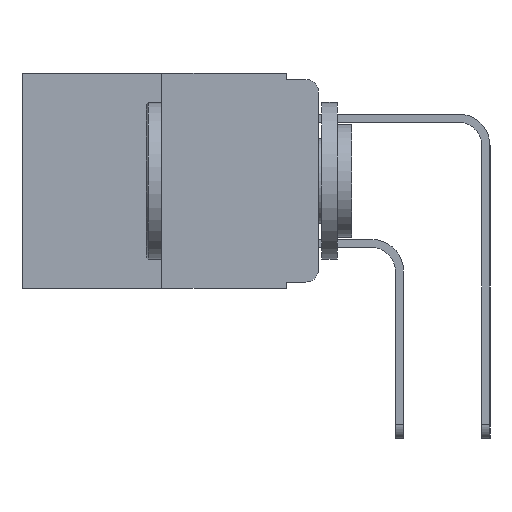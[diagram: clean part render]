
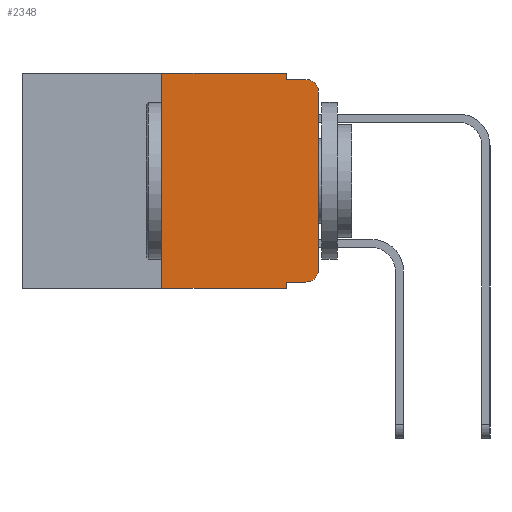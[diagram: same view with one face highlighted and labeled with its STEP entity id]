
A CAD part, left-side view. The second image highlights one B-rep face of the part: STEP entity #2348.
In plain terms, the highlighted planar face has unit normal (-1, 0, 0).
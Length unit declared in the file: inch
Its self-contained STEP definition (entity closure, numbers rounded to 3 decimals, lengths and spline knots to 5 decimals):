
#75 = ORIENTED_EDGE ( 'NONE', *, *, #12606, .F. ) ;
#532 = EDGE_CURVE ( 'NONE', #815, #10039, #12461, .T. ) ;
#646 = LINE ( 'NONE', #3511, #3547 ) ;
#777 = EDGE_CURVE ( 'NONE', #12841, #6741, #6242, .T. ) ;
#815 = VERTEX_POINT ( 'NONE', #12275 ) ;
#880 = AXIS2_PLACEMENT_3D ( 'NONE', #8151, #14173, #3209 ) ;
#946 = VECTOR ( 'NONE', #3475, 39.37008 ) ;
#975 = EDGE_LOOP ( 'NONE', ( #2216, #3295, #4586, #3999, #10049, #75, #2574, #1581, #1794, #2569 ) ) ;
#1115 = VERTEX_POINT ( 'NONE', #10265 ) ;
#1581 = ORIENTED_EDGE ( 'NONE', *, *, #7851, .F. ) ;
#1792 = CARTESIAN_POINT ( 'NONE',  ( 0., 0., -0.03 ) ) ;
#1794 = ORIENTED_EDGE ( 'NONE', *, *, #4811, .T. ) ;
#2216 = ORIENTED_EDGE ( 'NONE', *, *, #4131, .T. ) ;
#2348 = ADVANCED_FACE ( 'NONE', ( #10255 ), #11545, .F. ) ;
#2543 = CARTESIAN_POINT ( 'NONE',  ( 0., 0.051, -0.01 ) ) ;
#2569 = ORIENTED_EDGE ( 'NONE', *, *, #777, .T. ) ;
#2574 = ORIENTED_EDGE ( 'NONE', *, *, #11036, .T. ) ;
#2703 = VERTEX_POINT ( 'NONE', #3738 ) ;
#3000 = CARTESIAN_POINT ( 'NONE',  ( 0., 0.02, -0.313 ) ) ;
#3032 = DIRECTION ( 'NONE',  ( 0., 0., -1. ) ) ;
#3209 = DIRECTION ( 'NONE',  ( 0., 0., -1. ) ) ;
#3295 = ORIENTED_EDGE ( 'NONE', *, *, #5646, .T. ) ;
#3426 = VECTOR ( 'NONE', #4190, 39.37008 ) ;
#3443 = EDGE_CURVE ( 'NONE', #2703, #815, #9043, .T. ) ;
#3475 = DIRECTION ( 'NONE',  ( 0., 0., 1. ) ) ;
#3511 = CARTESIAN_POINT ( 'NONE',  ( 0., 0.473, 0. ) ) ;
#3547 = VECTOR ( 'NONE', #6862, 39.37008 ) ;
#3738 = CARTESIAN_POINT ( 'NONE',  ( 0., 0.051, 0. ) ) ;
#3834 = LINE ( 'NONE', #11164, #946 ) ;
#3999 = ORIENTED_EDGE ( 'NONE', *, *, #3443, .F. ) ;
#4131 = EDGE_CURVE ( 'NONE', #6741, #4433, #3834, .T. ) ;
#4190 = DIRECTION ( 'NONE',  ( 0., -1., 0. ) ) ;
#4214 = LINE ( 'NONE', #7473, #9705 ) ;
#4407 = AXIS2_PLACEMENT_3D ( 'NONE', #3000, #5075, #5576 ) ;
#4433 = VERTEX_POINT ( 'NONE', #1792 ) ;
#4586 = ORIENTED_EDGE ( 'NONE', *, *, #532, .F. ) ;
#4811 = EDGE_CURVE ( 'NONE', #12485, #12841, #6461, .T. ) ;
#4898 = CARTESIAN_POINT ( 'NONE',  ( 0., 0.051, -0.333 ) ) ;
#5075 = DIRECTION ( 'NONE',  ( -1., 0., 0. ) ) ;
#5100 = CARTESIAN_POINT ( 'NONE',  ( 0., 0.473, -0.343 ) ) ;
#5145 = VERTEX_POINT ( 'NONE', #11677 ) ;
#5342 = CARTESIAN_POINT ( 'NONE',  ( 0., 0.02, -0.333 ) ) ;
#5576 = DIRECTION ( 'NONE',  ( 0., 0., -1. ) ) ;
#5646 = EDGE_CURVE ( 'NONE', #4433, #10039, #8269, .T. ) ;
#6099 = CARTESIAN_POINT ( 'NONE',  ( 0., 0.25, -0.343 ) ) ;
#6230 = DIRECTION ( 'NONE',  ( -1., 0., 0. ) ) ;
#6233 = DIRECTION ( 'NONE',  ( 0., -1., 0. ) ) ;
#6242 = CIRCLE ( 'NONE', #4407, 0.02 ) ;
#6249 = LINE ( 'NONE', #5100, #11652 ) ;
#6461 = LINE ( 'NONE', #10736, #3426 ) ;
#6701 = EDGE_CURVE ( 'NONE', #5145, #2703, #646, .T. ) ;
#6741 = VERTEX_POINT ( 'NONE', #10165 ) ;
#6756 = VECTOR ( 'NONE', #7718, 39.37008 ) ;
#6862 = DIRECTION ( 'NONE',  ( 0., -1., 0. ) ) ;
#7215 = LINE ( 'NONE', #13698, #10089 ) ;
#7473 = CARTESIAN_POINT ( 'NONE',  ( 0., 0.051, 0. ) ) ;
#7718 = DIRECTION ( 'NONE',  ( 0., -1., 0. ) ) ;
#7851 = EDGE_CURVE ( 'NONE', #12485, #1115, #4214, .T. ) ;
#8151 = CARTESIAN_POINT ( 'NONE',  ( 0., 0.473, 0. ) ) ;
#8269 = CIRCLE ( 'NONE', #12304, 0.02 ) ;
#8704 = VECTOR ( 'NONE', #3032, 39.37008 ) ;
#9043 = LINE ( 'NONE', #10776, #8704 ) ;
#9705 = VECTOR ( 'NONE', #12802, 39.37008 ) ;
#10039 = VERTEX_POINT ( 'NONE', #11450 ) ;
#10049 = ORIENTED_EDGE ( 'NONE', *, *, #6701, .F. ) ;
#10089 = VECTOR ( 'NONE', #10521, 39.37008 ) ;
#10165 = CARTESIAN_POINT ( 'NONE',  ( 0., 0., -0.313 ) ) ;
#10255 = FACE_OUTER_BOUND ( 'NONE', #975, .T. ) ;
#10265 = CARTESIAN_POINT ( 'NONE',  ( 0., 0.051, -0.343 ) ) ;
#10521 = DIRECTION ( 'NONE',  ( 0., 0., 1. ) ) ;
#10736 = CARTESIAN_POINT ( 'NONE',  ( 0., 0.051, -0.333 ) ) ;
#10776 = CARTESIAN_POINT ( 'NONE',  ( 0., 0.051, 0. ) ) ;
#11036 = EDGE_CURVE ( 'NONE', #11698, #1115, #6249, .T. ) ;
#11164 = CARTESIAN_POINT ( 'NONE',  ( 0., 0., 0. ) ) ;
#11450 = CARTESIAN_POINT ( 'NONE',  ( 0., 0.02, -0.01 ) ) ;
#11545 = PLANE ( 'NONE',  #880 ) ;
#11652 = VECTOR ( 'NONE', #6233, 39.37008 ) ;
#11677 = CARTESIAN_POINT ( 'NONE',  ( 0., 0.25, 0. ) ) ;
#11698 = VERTEX_POINT ( 'NONE', #6099 ) ;
#12275 = CARTESIAN_POINT ( 'NONE',  ( 0., 0.051, -0.01 ) ) ;
#12304 = AXIS2_PLACEMENT_3D ( 'NONE', #12655, #6230, #13699 ) ;
#12461 = LINE ( 'NONE', #2543, #6756 ) ;
#12485 = VERTEX_POINT ( 'NONE', #4898 ) ;
#12606 = EDGE_CURVE ( 'NONE', #11698, #5145, #7215, .T. ) ;
#12655 = CARTESIAN_POINT ( 'NONE',  ( 0., 0.02, -0.03 ) ) ;
#12802 = DIRECTION ( 'NONE',  ( 0., 0., -1. ) ) ;
#12841 = VERTEX_POINT ( 'NONE', #5342 ) ;
#13698 = CARTESIAN_POINT ( 'NONE',  ( 0., 0.25, 0. ) ) ;
#13699 = DIRECTION ( 'NONE',  ( 0., 0., -1. ) ) ;
#14173 = DIRECTION ( 'NONE',  ( 1., 0., 0. ) ) ;
